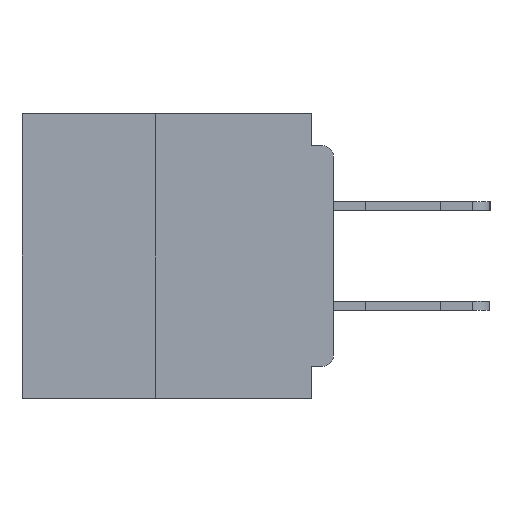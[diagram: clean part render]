
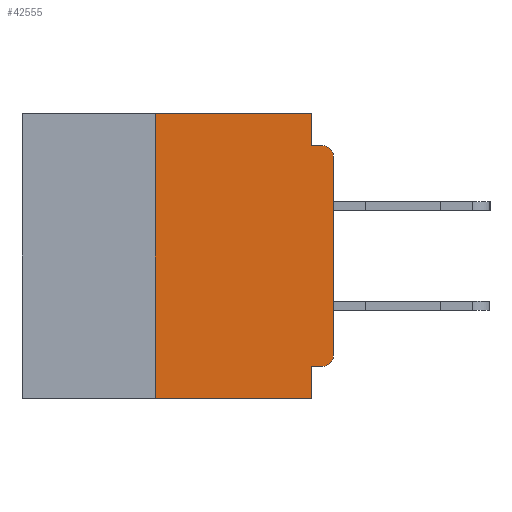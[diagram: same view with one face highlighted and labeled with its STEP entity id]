
A CAD part, left-side view. The second image highlights one B-rep face of the part: STEP entity #42555.
In plain terms, the highlighted planar face has unit normal (-1, 0, 0).
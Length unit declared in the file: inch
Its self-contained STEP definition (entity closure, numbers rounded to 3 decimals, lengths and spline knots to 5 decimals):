
#458 = VERTEX_POINT ( 'NONE', #21426 ) ;
#552 = DIRECTION ( 'NONE',  ( 0., 0., -1. ) ) ;
#1930 = VERTEX_POINT ( 'NONE', #18767 ) ;
#2243 = CARTESIAN_POINT ( 'NONE',  ( 0., 0.25, 0. ) ) ;
#4273 = EDGE_CURVE ( 'NONE', #39063, #29013, #18596, .T. ) ;
#5344 = EDGE_CURVE ( 'NONE', #41089, #458, #31907, .T. ) ;
#6060 = ORIENTED_EDGE ( 'NONE', *, *, #52669, .F. ) ;
#6085 = LINE ( 'NONE', #48418, #51187 ) ;
#6762 = ORIENTED_EDGE ( 'NONE', *, *, #5344, .F. ) ;
#6918 = CARTESIAN_POINT ( 'NONE',  ( 0., 0., -0.06 ) ) ;
#7129 = DIRECTION ( 'NONE',  ( 0., -1., 0. ) ) ;
#8038 = CARTESIAN_POINT ( 'NONE',  ( 0., 0.031, -0.355 ) ) ;
#8164 = ORIENTED_EDGE ( 'NONE', *, *, #19293, .F. ) ;
#8314 = LINE ( 'NONE', #27564, #18884 ) ;
#8379 = CARTESIAN_POINT ( 'NONE',  ( 0., 0.437, -0.4 ) ) ;
#10399 = VERTEX_POINT ( 'NONE', #29010 ) ;
#10789 = AXIS2_PLACEMENT_3D ( 'NONE', #31271, #53689, #40337 ) ;
#11085 = DIRECTION ( 'NONE',  ( 0., 0., -1. ) ) ;
#11920 = CARTESIAN_POINT ( 'NONE',  ( 0., 0., 0. ) ) ;
#11948 = CARTESIAN_POINT ( 'NONE',  ( 0., 0., -0.34 ) ) ;
#13622 = DIRECTION ( 'NONE',  ( 0., 0., 1. ) ) ;
#13626 = EDGE_CURVE ( 'NONE', #10399, #41159, #16615, .T. ) ;
#15069 = LINE ( 'NONE', #42553, #39019 ) ;
#16615 = CIRCLE ( 'NONE', #55628, 0.015 ) ;
#16981 = VERTEX_POINT ( 'NONE', #55864 ) ;
#17364 = ORIENTED_EDGE ( 'NONE', *, *, #20701, .F. ) ;
#17564 = LINE ( 'NONE', #11920, #29526 ) ;
#17796 = EDGE_CURVE ( 'NONE', #41159, #39063, #17564, .T. ) ;
#18596 = CIRCLE ( 'NONE', #49261, 0.015 ) ;
#18767 = CARTESIAN_POINT ( 'NONE',  ( 0., 0.031, -0.045 ) ) ;
#18884 = VECTOR ( 'NONE', #552, 39.37008 ) ;
#19293 = EDGE_CURVE ( 'NONE', #48424, #41089, #32418, .T. ) ;
#19962 = VECTOR ( 'NONE', #23189, 39.37008 ) ;
#20516 = CARTESIAN_POINT ( 'NONE',  ( 0., 0., -0.045 ) ) ;
#20701 = EDGE_CURVE ( 'NONE', #458, #1930, #8314, .T. ) ;
#21426 = CARTESIAN_POINT ( 'NONE',  ( 0., 0.031, 0. ) ) ;
#21507 = CARTESIAN_POINT ( 'NONE',  ( 0., 0.015, -0.34 ) ) ;
#23189 = DIRECTION ( 'NONE',  ( 0., -1., 0. ) ) ;
#23308 = CARTESIAN_POINT ( 'NONE',  ( 0., 0.437, 0. ) ) ;
#23670 = ORIENTED_EDGE ( 'NONE', *, *, #4273, .T. ) ;
#24091 = VECTOR ( 'NONE', #7129, 39.37008 ) ;
#26022 = DIRECTION ( 'NONE',  ( 0., 0., -1. ) ) ;
#27564 = CARTESIAN_POINT ( 'NONE',  ( 0., 0.031, 0. ) ) ;
#28592 = ORIENTED_EDGE ( 'NONE', *, *, #33550, .F. ) ;
#29010 = CARTESIAN_POINT ( 'NONE',  ( 0., 0.015, -0.355 ) ) ;
#29013 = VERTEX_POINT ( 'NONE', #37379 ) ;
#29526 = VECTOR ( 'NONE', #34382, 39.37008 ) ;
#30041 = ORIENTED_EDGE ( 'NONE', *, *, #13626, .T. ) ;
#31271 = CARTESIAN_POINT ( 'NONE',  ( 0., 0.437, 0. ) ) ;
#31381 = ORIENTED_EDGE ( 'NONE', *, *, #17796, .T. ) ;
#31907 = LINE ( 'NONE', #23308, #19962 ) ;
#32418 = LINE ( 'NONE', #54130, #33867 ) ;
#32523 = VECTOR ( 'NONE', #39910, 39.37008 ) ;
#33550 = EDGE_CURVE ( 'NONE', #58257, #16981, #15069, .T. ) ;
#33867 = VECTOR ( 'NONE', #13622, 39.37008 ) ;
#34382 = DIRECTION ( 'NONE',  ( 0., 0., 1. ) ) ;
#34982 = ORIENTED_EDGE ( 'NONE', *, *, #55218, .T. ) ;
#35659 = ORIENTED_EDGE ( 'NONE', *, *, #50656, .F. ) ;
#35838 = PLANE ( 'NONE',  #10789 ) ;
#36069 = LINE ( 'NONE', #20516, #24091 ) ;
#37133 = DIRECTION ( 'NONE',  ( -1., 0., 0. ) ) ;
#37140 = DIRECTION ( 'NONE',  ( 0., 0., -1. ) ) ;
#37327 = CARTESIAN_POINT ( 'NONE',  ( 0., 0.015, -0.06 ) ) ;
#37379 = CARTESIAN_POINT ( 'NONE',  ( 0., 0.015, -0.045 ) ) ;
#38366 = FACE_OUTER_BOUND ( 'NONE', #39500, .T. ) ;
#39019 = VECTOR ( 'NONE', #11085, 39.37008 ) ;
#39063 = VERTEX_POINT ( 'NONE', #6918 ) ;
#39500 = EDGE_LOOP ( 'NONE', ( #31381, #23670, #35659, #17364, #6762, #8164, #34982, #28592, #6060, #30041 ) ) ;
#39910 = DIRECTION ( 'NONE',  ( 0., -1., 0. ) ) ;
#40337 = DIRECTION ( 'NONE',  ( 0., 0., -1. ) ) ;
#41089 = VERTEX_POINT ( 'NONE', #2243 ) ;
#41159 = VERTEX_POINT ( 'NONE', #11948 ) ;
#42553 = CARTESIAN_POINT ( 'NONE',  ( 0., 0.031, -0.4 ) ) ;
#42555 = ADVANCED_FACE ( 'NONE', ( #38366 ), #35838, .F. ) ;
#43103 = LINE ( 'NONE', #8379, #32523 ) ;
#48418 = CARTESIAN_POINT ( 'NONE',  ( 0., 0., -0.355 ) ) ;
#48424 = VERTEX_POINT ( 'NONE', #54942 ) ;
#49261 = AXIS2_PLACEMENT_3D ( 'NONE', #37327, #37133, #37140 ) ;
#50656 = EDGE_CURVE ( 'NONE', #1930, #29013, #36069, .T. ) ;
#51187 = VECTOR ( 'NONE', #52758, 39.37008 ) ;
#52669 = EDGE_CURVE ( 'NONE', #10399, #58257, #6085, .T. ) ;
#52758 = DIRECTION ( 'NONE',  ( 0., 1., 0. ) ) ;
#52955 = DIRECTION ( 'NONE',  ( -1., 0., 0. ) ) ;
#53689 = DIRECTION ( 'NONE',  ( 1., 0., 0. ) ) ;
#54130 = CARTESIAN_POINT ( 'NONE',  ( 0., 0.25, -0.4 ) ) ;
#54942 = CARTESIAN_POINT ( 'NONE',  ( 0., 0.25, -0.4 ) ) ;
#55218 = EDGE_CURVE ( 'NONE', #48424, #16981, #43103, .T. ) ;
#55628 = AXIS2_PLACEMENT_3D ( 'NONE', #21507, #52955, #26022 ) ;
#55864 = CARTESIAN_POINT ( 'NONE',  ( 0., 0.031, -0.4 ) ) ;
#58257 = VERTEX_POINT ( 'NONE', #8038 ) ;
